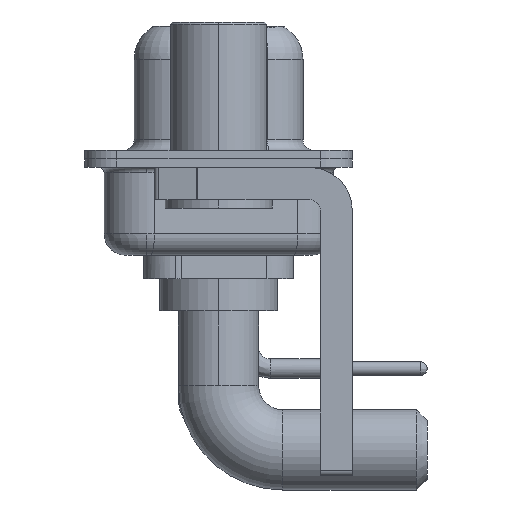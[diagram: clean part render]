
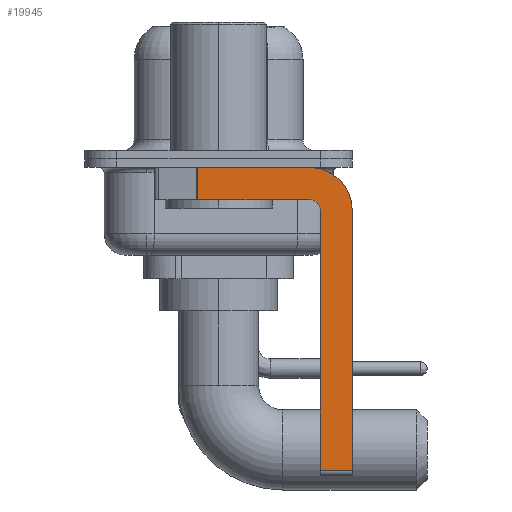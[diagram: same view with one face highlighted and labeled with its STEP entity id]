
A CAD part, left-side view. The second image highlights one B-rep face of the part: STEP entity #19945.
In plain terms, the highlighted planar face has unit normal (-1, 0, 0).
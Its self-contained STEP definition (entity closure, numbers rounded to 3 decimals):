
#532 = CARTESIAN_POINT ( 'NONE',  ( -2.9, -4.25, -0.4 ) ) ;
#929 = CARTESIAN_POINT ( 'NONE',  ( -2.9, -4.25, -1.9 ) ) ;
#992 = EDGE_CURVE ( 'NONE', #9428, #4455, #5955, .T. ) ;
#1219 = CARTESIAN_POINT ( 'NONE',  ( -2.9, -4.25, -2.4 ) ) ;
#1333 = EDGE_LOOP ( 'NONE', ( #14991, #11737, #8663, #2823, #12795, #10054, #11193, #9446 ) ) ;
#1335 = DIRECTION ( 'NONE',  ( 0., 0., -1. ) ) ;
#1382 = DIRECTION ( 'NONE',  ( 0., 0., -1. ) ) ;
#1437 = DIRECTION ( 'NONE',  ( 1., 0., 0. ) ) ;
#2229 = VERTEX_POINT ( 'NONE', #17960 ) ;
#2823 = ORIENTED_EDGE ( 'NONE', *, *, #14780, .F. ) ;
#3392 = CARTESIAN_POINT ( 'NONE',  ( -2.9, -4.25, -2.4 ) ) ;
#3625 = CARTESIAN_POINT ( 'NONE',  ( -2.9, 3., -0.4 ) ) ;
#3760 = EDGE_CURVE ( 'NONE', #9428, #8174, #16442, .T. ) ;
#4455 = VERTEX_POINT ( 'NONE', #5085 ) ;
#4590 = CARTESIAN_POINT ( 'NONE',  ( -2.9, -4.25, -2.4 ) ) ;
#4741 = CARTESIAN_POINT ( 'NONE',  ( -2.9, -4.25, -14.55 ) ) ;
#4809 = DIRECTION ( 'NONE',  ( 1., 0., 0. ) ) ;
#4812 = PLANE ( 'NONE',  #5802 ) ;
#5085 = CARTESIAN_POINT ( 'NONE',  ( -2.9, -6.25, -14.55 ) ) ;
#5268 = LINE ( 'NONE', #3625, #17344 ) ;
#5637 = VERTEX_POINT ( 'NONE', #532 ) ;
#5802 = AXIS2_PLACEMENT_3D ( 'NONE', #3392, #1437, #1335 ) ;
#5955 = LINE ( 'NONE', #4741, #10122 ) ;
#6270 = VERTEX_POINT ( 'NONE', #929 ) ;
#6836 = LINE ( 'NONE', #20897, #8945 ) ;
#7820 = CIRCLE ( 'NONE', #10594, 0.5 ) ;
#8035 = AXIS2_PLACEMENT_3D ( 'NONE', #1219, #4809, #11445 ) ;
#8172 = EDGE_CURVE ( 'NONE', #15328, #4455, #9708, .T. ) ;
#8174 = VERTEX_POINT ( 'NONE', #17597 ) ;
#8329 = VECTOR ( 'NONE', #10916, 1000. ) ;
#8663 = ORIENTED_EDGE ( 'NONE', *, *, #17464, .F. ) ;
#8945 = VECTOR ( 'NONE', #20168, 1000. ) ;
#9428 = VERTEX_POINT ( 'NONE', #15728 ) ;
#9446 = ORIENTED_EDGE ( 'NONE', *, *, #9467, .F. ) ;
#9467 = EDGE_CURVE ( 'NONE', #5637, #15328, #13946, .T. ) ;
#9708 = LINE ( 'NONE', #21403, #8329 ) ;
#9782 = DIRECTION ( 'NONE',  ( 0., 0., 1. ) ) ;
#10054 = ORIENTED_EDGE ( 'NONE', *, *, #992, .T. ) ;
#10122 = VECTOR ( 'NONE', #11384, 1000. ) ;
#10272 = DIRECTION ( 'NONE',  ( 0., -1., 0. ) ) ;
#10345 = EDGE_CURVE ( 'NONE', #19227, #2229, #21258, .T. ) ;
#10594 = AXIS2_PLACEMENT_3D ( 'NONE', #4590, #13166, #18122 ) ;
#10916 = DIRECTION ( 'NONE',  ( 0., 0., -1. ) ) ;
#11193 = ORIENTED_EDGE ( 'NONE', *, *, #8172, .F. ) ;
#11199 = CARTESIAN_POINT ( 'NONE',  ( -2.9, 0.978, -1.9 ) ) ;
#11384 = DIRECTION ( 'NONE',  ( 0., -1., 0. ) ) ;
#11445 = DIRECTION ( 'NONE',  ( 0., 0., -1. ) ) ;
#11737 = ORIENTED_EDGE ( 'NONE', *, *, #10345, .T. ) ;
#12340 = FACE_OUTER_BOUND ( 'NONE', #1333, .T. ) ;
#12539 = CARTESIAN_POINT ( 'NONE',  ( -2.9, -6.25, -2.4 ) ) ;
#12793 = VECTOR ( 'NONE', #9782, 1000. ) ;
#12795 = ORIENTED_EDGE ( 'NONE', *, *, #3760, .F. ) ;
#13166 = DIRECTION ( 'NONE',  ( -1., 0., 0. ) ) ;
#13946 = CIRCLE ( 'NONE', #8035, 2. ) ;
#14780 = EDGE_CURVE ( 'NONE', #8174, #6270, #7820, .T. ) ;
#14991 = ORIENTED_EDGE ( 'NONE', *, *, #17861, .F. ) ;
#15328 = VERTEX_POINT ( 'NONE', #12539 ) ;
#15728 = CARTESIAN_POINT ( 'NONE',  ( -2.9, -4.75, -14.55 ) ) ;
#16442 = LINE ( 'NONE', #19728, #12793 ) ;
#16767 = VECTOR ( 'NONE', #1382, 1000. ) ;
#17344 = VECTOR ( 'NONE', #10272, 1000. ) ;
#17464 = EDGE_CURVE ( 'NONE', #6270, #2229, #6836, .T. ) ;
#17597 = CARTESIAN_POINT ( 'NONE',  ( -2.9, -4.75, -2.4 ) ) ;
#17861 = EDGE_CURVE ( 'NONE', #19227, #5637, #5268, .T. ) ;
#17960 = CARTESIAN_POINT ( 'NONE',  ( -2.9, 0.978, -1.9 ) ) ;
#18122 = DIRECTION ( 'NONE',  ( 0., 0., 1. ) ) ;
#19227 = VERTEX_POINT ( 'NONE', #19742 ) ;
#19728 = CARTESIAN_POINT ( 'NONE',  ( -2.9, -4.75, -14.8 ) ) ;
#19742 = CARTESIAN_POINT ( 'NONE',  ( -2.9, 0.978, -0.4 ) ) ;
#19945 = ADVANCED_FACE ( 'NONE', ( #12340 ), #4812, .F. ) ;
#20168 = DIRECTION ( 'NONE',  ( 0., 1., 0. ) ) ;
#20897 = CARTESIAN_POINT ( 'NONE',  ( -2.9, -4.25, -1.9 ) ) ;
#21258 = LINE ( 'NONE', #11199, #16767 ) ;
#21403 = CARTESIAN_POINT ( 'NONE',  ( -2.9, -6.25, -2.4 ) ) ;
